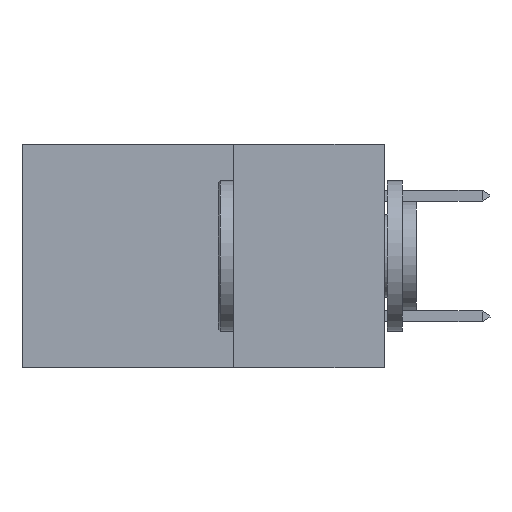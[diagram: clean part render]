
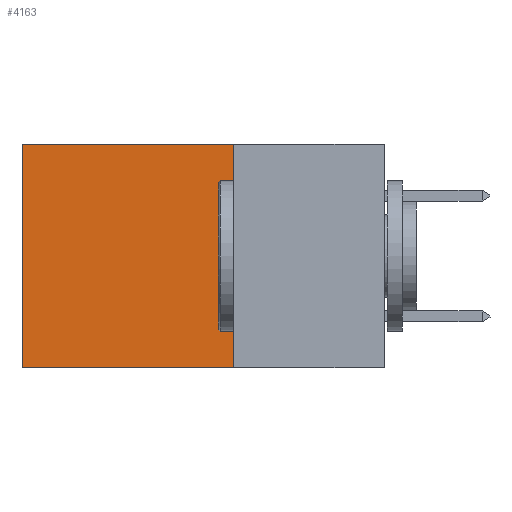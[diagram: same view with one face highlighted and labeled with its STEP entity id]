
A CAD part, left-side view. The second image highlights one B-rep face of the part: STEP entity #4163.
In plain terms, the highlighted planar face has unit normal (-1, 0, 0).
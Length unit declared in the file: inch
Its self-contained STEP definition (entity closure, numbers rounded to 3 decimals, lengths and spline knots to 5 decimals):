
#756 = CARTESIAN_POINT ( 'NONE',  ( 0.2875, 0.25, -0.37 ) ) ;
#757 = CARTESIAN_POINT ( 'NONE',  ( 0.2875, 0.25, 0. ) ) ;
#812 = LINE ( 'NONE', #6280, #12473 ) ;
#1360 = DIRECTION ( 'NONE',  ( 0., 1., 0. ) ) ;
#1933 = EDGE_CURVE ( 'NONE', #12324, #8974, #10755, .T. ) ;
#3339 = ORIENTED_EDGE ( 'NONE', *, *, #9789, .T. ) ;
#4163 = ADVANCED_FACE ( 'NONE', ( #11535 ), #13750, .F. ) ;
#4191 = ORIENTED_EDGE ( 'NONE', *, *, #18127, .F. ) ;
#5131 = CARTESIAN_POINT ( 'NONE',  ( 0.2875, 0.6, -0.37 ) ) ;
#5307 = AXIS2_PLACEMENT_3D ( 'NONE', #13478, #13730, #18648 ) ;
#6280 = CARTESIAN_POINT ( 'NONE',  ( 0.2875, 0.25, 0. ) ) ;
#7828 = DIRECTION ( 'NONE',  ( 0., 1., 0. ) ) ;
#7935 = CARTESIAN_POINT ( 'NONE',  ( 0.2875, 0.25, 0. ) ) ;
#8078 = VECTOR ( 'NONE', #15820, 39.37008 ) ;
#8643 = ORIENTED_EDGE ( 'NONE', *, *, #10177, .T. ) ;
#8867 = VERTEX_POINT ( 'NONE', #7935 ) ;
#8974 = VERTEX_POINT ( 'NONE', #5131 ) ;
#9662 = ORIENTED_EDGE ( 'NONE', *, *, #1933, .F. ) ;
#9789 = EDGE_CURVE ( 'NONE', #17374, #8974, #16421, .T. ) ;
#10177 = EDGE_CURVE ( 'NONE', #8867, #17374, #812, .T. ) ;
#10277 = CARTESIAN_POINT ( 'NONE',  ( 0.2875, 0.25, -0.37 ) ) ;
#10669 = EDGE_LOOP ( 'NONE', ( #3339, #9662, #4191, #8643 ) ) ;
#10755 = LINE ( 'NONE', #756, #18084 ) ;
#11535 = FACE_OUTER_BOUND ( 'NONE', #10669, .T. ) ;
#12324 = VERTEX_POINT ( 'NONE', #10277 ) ;
#12473 = VECTOR ( 'NONE', #7828, 39.37008 ) ;
#13478 = CARTESIAN_POINT ( 'NONE',  ( 0.2875, 0.25, 0. ) ) ;
#13730 = DIRECTION ( 'NONE',  ( 1., 0., 0. ) ) ;
#13750 = PLANE ( 'NONE',  #5307 ) ;
#14171 = VECTOR ( 'NONE', #17326, 39.37008 ) ;
#14381 = CARTESIAN_POINT ( 'NONE',  ( 0.2875, 0.6, 0. ) ) ;
#15481 = CARTESIAN_POINT ( 'NONE',  ( 0.2875, 0.6, 0. ) ) ;
#15820 = DIRECTION ( 'NONE',  ( 0., 0., -1. ) ) ;
#16421 = LINE ( 'NONE', #14381, #8078 ) ;
#17326 = DIRECTION ( 'NONE',  ( 0., 0., -1. ) ) ;
#17374 = VERTEX_POINT ( 'NONE', #15481 ) ;
#18084 = VECTOR ( 'NONE', #1360, 39.37008 ) ;
#18127 = EDGE_CURVE ( 'NONE', #8867, #12324, #18981, .T. ) ;
#18648 = DIRECTION ( 'NONE',  ( 0., 0., -1. ) ) ;
#18981 = LINE ( 'NONE', #757, #14171 ) ;
